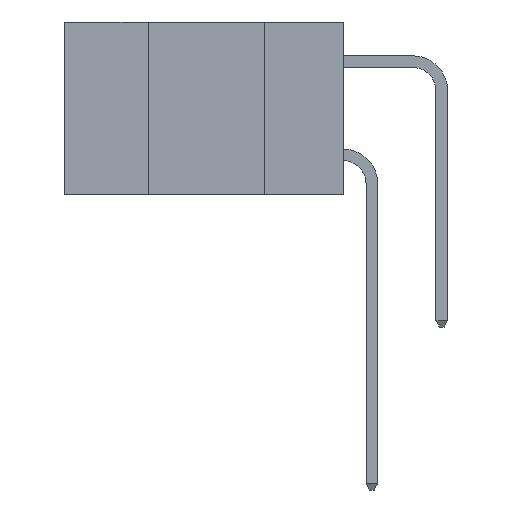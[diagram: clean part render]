
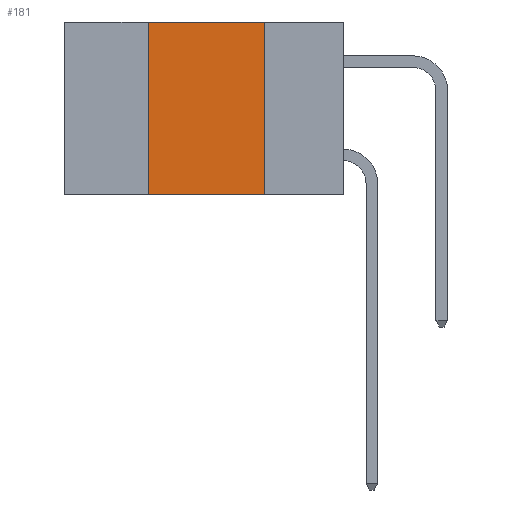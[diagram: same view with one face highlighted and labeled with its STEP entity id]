
A CAD part, left-side view. The second image highlights one B-rep face of the part: STEP entity #181.
In plain terms, the highlighted planar face has unit normal (-1, 0, 0).
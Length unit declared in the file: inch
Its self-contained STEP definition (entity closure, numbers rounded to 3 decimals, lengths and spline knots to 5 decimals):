
#170 = EDGE_CURVE ( 'NONE', #11916, #10671, #5442, .T. ) ;
#181 = ADVANCED_FACE ( 'NONE', ( #7934 ), #10549, .F. ) ;
#364 = CARTESIAN_POINT ( 'NONE',  ( 0., 0.17, -0.37 ) ) ;
#1257 = VERTEX_POINT ( 'NONE', #364 ) ;
#1334 = VECTOR ( 'NONE', #3886, 39.37008 ) ;
#1464 = AXIS2_PLACEMENT_3D ( 'NONE', #10247, #10447, #9055 ) ;
#1756 = CARTESIAN_POINT ( 'NONE',  ( 0., 0.42, 0. ) ) ;
#1953 = EDGE_CURVE ( 'NONE', #10671, #1257, #7197, .T. ) ;
#3492 = CARTESIAN_POINT ( 'NONE',  ( 0., 0.42, -0.37 ) ) ;
#3886 = DIRECTION ( 'NONE',  ( 0., 0., -1. ) ) ;
#4031 = VECTOR ( 'NONE', #6955, 39.37008 ) ;
#4892 = DIRECTION ( 'NONE',  ( 0., 0., 1. ) ) ;
#5442 = LINE ( 'NONE', #10462, #10783 ) ;
#5933 = CARTESIAN_POINT ( 'NONE',  ( 0., 0.42, -0.37 ) ) ;
#6935 = LINE ( 'NONE', #5933, #11961 ) ;
#6955 = DIRECTION ( 'NONE',  ( 0., -1., 0. ) ) ;
#7021 = CARTESIAN_POINT ( 'NONE',  ( 0., 0.17, -0.37 ) ) ;
#7026 = ORIENTED_EDGE ( 'NONE', *, *, #1953, .F. ) ;
#7197 = LINE ( 'NONE', #7021, #1334 ) ;
#7214 = ORIENTED_EDGE ( 'NONE', *, *, #170, .F. ) ;
#7934 = FACE_OUTER_BOUND ( 'NONE', #10877, .T. ) ;
#8218 = ORIENTED_EDGE ( 'NONE', *, *, #13985, .F. ) ;
#9055 = DIRECTION ( 'NONE',  ( 0., 0., -1. ) ) ;
#9186 = CARTESIAN_POINT ( 'NONE',  ( 0., 0.6, -0.37 ) ) ;
#10247 = CARTESIAN_POINT ( 'NONE',  ( 0., 0.6, 0. ) ) ;
#10447 = DIRECTION ( 'NONE',  ( 1., 0., 0. ) ) ;
#10462 = CARTESIAN_POINT ( 'NONE',  ( 0., 0.6, 0. ) ) ;
#10488 = DIRECTION ( 'NONE',  ( 0., -1., 0. ) ) ;
#10549 = PLANE ( 'NONE',  #1464 ) ;
#10671 = VERTEX_POINT ( 'NONE', #11775 ) ;
#10783 = VECTOR ( 'NONE', #10488, 39.37008 ) ;
#10877 = EDGE_LOOP ( 'NONE', ( #7026, #7214, #8218, #10898 ) ) ;
#10898 = ORIENTED_EDGE ( 'NONE', *, *, #13948, .T. ) ;
#11702 = VERTEX_POINT ( 'NONE', #3492 ) ;
#11775 = CARTESIAN_POINT ( 'NONE',  ( 0., 0.17, 0. ) ) ;
#11916 = VERTEX_POINT ( 'NONE', #1756 ) ;
#11961 = VECTOR ( 'NONE', #4892, 39.37008 ) ;
#12631 = LINE ( 'NONE', #9186, #4031 ) ;
#13948 = EDGE_CURVE ( 'NONE', #11702, #1257, #12631, .T. ) ;
#13985 = EDGE_CURVE ( 'NONE', #11702, #11916, #6935, .T. ) ;
